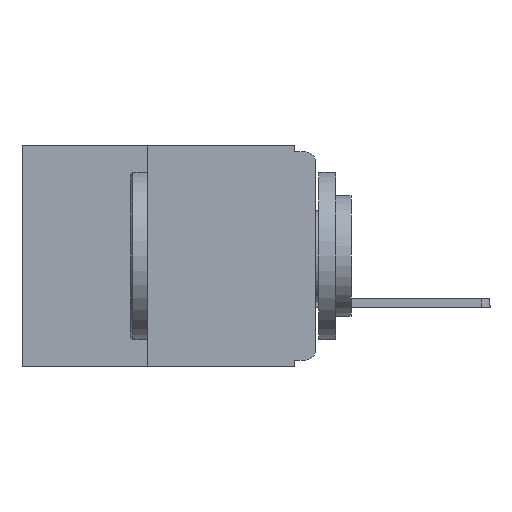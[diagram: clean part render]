
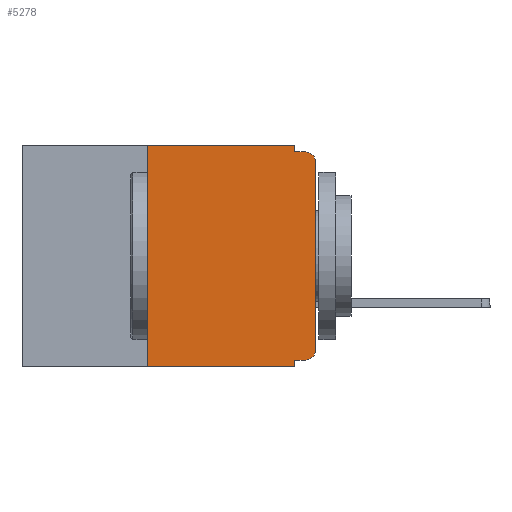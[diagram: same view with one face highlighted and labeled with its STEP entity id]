
A CAD part, left-side view. The second image highlights one B-rep face of the part: STEP entity #5278.
In plain terms, the highlighted planar face has unit normal (-1, 0, 0).
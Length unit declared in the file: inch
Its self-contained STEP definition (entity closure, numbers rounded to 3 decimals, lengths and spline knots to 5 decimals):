
#703 = VERTEX_POINT ( 'NONE', #7214 ) ;
#1184 = CARTESIAN_POINT ( 'NONE',  ( 0., 0., -0.32 ) ) ;
#1362 = DIRECTION ( 'NONE',  ( 0., 0., -1. ) ) ;
#1621 = CARTESIAN_POINT ( 'NONE',  ( 0., 0., -0.305 ) ) ;
#1974 = VECTOR ( 'NONE', #15401, 39.37008 ) ;
#2550 = DIRECTION ( 'NONE',  ( 0., 0., -1. ) ) ;
#3487 = ORIENTED_EDGE ( 'NONE', *, *, #4456, .T. ) ;
#3526 = DIRECTION ( 'NONE',  ( 0., -1., 0. ) ) ;
#4456 = EDGE_CURVE ( 'NONE', #19598, #15217, #19629, .T. ) ;
#4556 = EDGE_CURVE ( 'NONE', #7260, #19598, #17381, .T. ) ;
#4559 = AXIS2_PLACEMENT_3D ( 'NONE', #5997, #5968, #5911 ) ;
#5278 = ADVANCED_FACE ( 'NONE', ( #11664 ), #22277, .F. ) ;
#5656 = VERTEX_POINT ( 'NONE', #7245 ) ;
#5711 = ORIENTED_EDGE ( 'NONE', *, *, #16454, .F. ) ;
#5911 = DIRECTION ( 'NONE',  ( 0., 0., -1. ) ) ;
#5968 = DIRECTION ( 'NONE',  ( -1., 0., 0. ) ) ;
#5997 = CARTESIAN_POINT ( 'NONE',  ( 0., 0.015, -0.305 ) ) ;
#6127 = VECTOR ( 'NONE', #6564, 39.37008 ) ;
#6154 = CARTESIAN_POINT ( 'NONE',  ( 0., 0.015, -0.32 ) ) ;
#6174 = VECTOR ( 'NONE', #15181, 39.37008 ) ;
#6292 = ORIENTED_EDGE ( 'NONE', *, *, #20045, .F. ) ;
#6564 = DIRECTION ( 'NONE',  ( 0., 1., 0. ) ) ;
#7214 = CARTESIAN_POINT ( 'NONE',  ( 0., 0.031, -0.01 ) ) ;
#7245 = CARTESIAN_POINT ( 'NONE',  ( 0., 0.031, -0.32 ) ) ;
#7260 = VERTEX_POINT ( 'NONE', #6154 ) ;
#7385 = EDGE_CURVE ( 'NONE', #15217, #14455, #11875, .T. ) ;
#7587 = CARTESIAN_POINT ( 'NONE',  ( 0., 0., 0. ) ) ;
#7641 = DIRECTION ( 'NONE',  ( 0., 0., 1. ) ) ;
#7857 = DIRECTION ( 'NONE',  ( 0., -1., 0. ) ) ;
#8046 = LINE ( 'NONE', #11896, #20197 ) ;
#8213 = CARTESIAN_POINT ( 'NONE',  ( 0., 0.25, -0.33 ) ) ;
#8251 = ORIENTED_EDGE ( 'NONE', *, *, #7385, .T. ) ;
#8350 = DIRECTION ( 'NONE',  ( -1., 0., 0. ) ) ;
#8513 = VECTOR ( 'NONE', #7857, 39.37008 ) ;
#8532 = EDGE_CURVE ( 'NONE', #19978, #17535, #15787, .T. ) ;
#8968 = AXIS2_PLACEMENT_3D ( 'NONE', #19196, #8350, #20958 ) ;
#9975 = EDGE_CURVE ( 'NONE', #703, #14455, #11041, .T. ) ;
#10086 = CARTESIAN_POINT ( 'NONE',  ( 0., 0.25, 0. ) ) ;
#10452 = VECTOR ( 'NONE', #3526, 39.37008 ) ;
#10781 = VERTEX_POINT ( 'NONE', #10086 ) ;
#11041 = LINE ( 'NONE', #17896, #10452 ) ;
#11108 = ORIENTED_EDGE ( 'NONE', *, *, #4556, .T. ) ;
#11291 = VERTEX_POINT ( 'NONE', #11553 ) ;
#11553 = CARTESIAN_POINT ( 'NONE',  ( 0., 0.031, 0. ) ) ;
#11664 = FACE_OUTER_BOUND ( 'NONE', #14407, .T. ) ;
#11668 = CARTESIAN_POINT ( 'NONE',  ( 0., 0.031, -0.33 ) ) ;
#11875 = CIRCLE ( 'NONE', #8968, 0.015 ) ;
#11896 = CARTESIAN_POINT ( 'NONE',  ( 0., 0.25, -0.33 ) ) ;
#12144 = LINE ( 'NONE', #22515, #1974 ) ;
#12496 = CARTESIAN_POINT ( 'NONE',  ( 0., 0.015, -0.01 ) ) ;
#12579 = EDGE_CURVE ( 'NONE', #19978, #10781, #8046, .T. ) ;
#13342 = DIRECTION ( 'NONE',  ( 1., 0., 0. ) ) ;
#13408 = CARTESIAN_POINT ( 'NONE',  ( 0., 0., -0.025 ) ) ;
#14291 = VECTOR ( 'NONE', #7641, 39.37008 ) ;
#14407 = EDGE_LOOP ( 'NONE', ( #3487, #8251, #22600, #23150, #19016, #14788, #19575, #5711, #6292, #11108 ) ) ;
#14455 = VERTEX_POINT ( 'NONE', #12496 ) ;
#14788 = ORIENTED_EDGE ( 'NONE', *, *, #12579, .F. ) ;
#15092 = VECTOR ( 'NONE', #1362, 39.37008 ) ;
#15181 = DIRECTION ( 'NONE',  ( 0., -1., 0. ) ) ;
#15217 = VERTEX_POINT ( 'NONE', #13408 ) ;
#15401 = DIRECTION ( 'NONE',  ( 0., 0., -1. ) ) ;
#15638 = LINE ( 'NONE', #22933, #15092 ) ;
#15787 = LINE ( 'NONE', #17003, #6174 ) ;
#16454 = EDGE_CURVE ( 'NONE', #5656, #17535, #15638, .T. ) ;
#16987 = AXIS2_PLACEMENT_3D ( 'NONE', #20514, #13342, #2550 ) ;
#17003 = CARTESIAN_POINT ( 'NONE',  ( 0., 0.437, -0.33 ) ) ;
#17381 = CIRCLE ( 'NONE', #4559, 0.015 ) ;
#17535 = VERTEX_POINT ( 'NONE', #11668 ) ;
#17896 = CARTESIAN_POINT ( 'NONE',  ( 0., 0., -0.01 ) ) ;
#18146 = LINE ( 'NONE', #20481, #8513 ) ;
#19016 = ORIENTED_EDGE ( 'NONE', *, *, #21116, .F. ) ;
#19196 = CARTESIAN_POINT ( 'NONE',  ( 0., 0.015, -0.025 ) ) ;
#19575 = ORIENTED_EDGE ( 'NONE', *, *, #8532, .T. ) ;
#19598 = VERTEX_POINT ( 'NONE', #1621 ) ;
#19629 = LINE ( 'NONE', #7587, #14291 ) ;
#19978 = VERTEX_POINT ( 'NONE', #8213 ) ;
#20045 = EDGE_CURVE ( 'NONE', #7260, #5656, #20523, .T. ) ;
#20197 = VECTOR ( 'NONE', #21023, 39.37008 ) ;
#20481 = CARTESIAN_POINT ( 'NONE',  ( 0., 0.437, 0. ) ) ;
#20514 = CARTESIAN_POINT ( 'NONE',  ( 0., 0.437, 0. ) ) ;
#20523 = LINE ( 'NONE', #1184, #6127 ) ;
#20958 = DIRECTION ( 'NONE',  ( 0., 0., -1. ) ) ;
#21023 = DIRECTION ( 'NONE',  ( 0., 0., 1. ) ) ;
#21116 = EDGE_CURVE ( 'NONE', #10781, #11291, #18146, .T. ) ;
#22034 = EDGE_CURVE ( 'NONE', #11291, #703, #12144, .T. ) ;
#22277 = PLANE ( 'NONE',  #16987 ) ;
#22515 = CARTESIAN_POINT ( 'NONE',  ( 0., 0.031, 0. ) ) ;
#22600 = ORIENTED_EDGE ( 'NONE', *, *, #9975, .F. ) ;
#22933 = CARTESIAN_POINT ( 'NONE',  ( 0., 0.031, -0.33 ) ) ;
#23150 = ORIENTED_EDGE ( 'NONE', *, *, #22034, .F. ) ;
